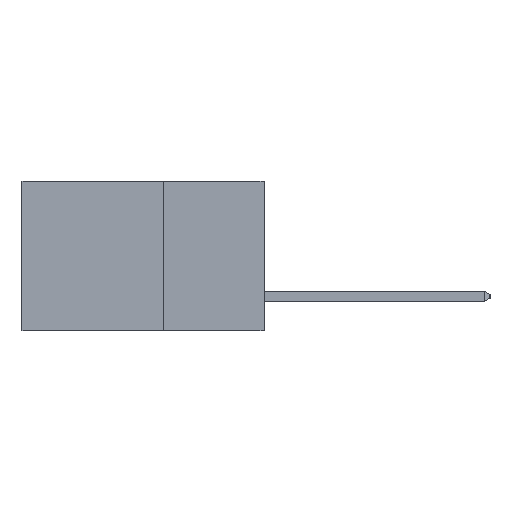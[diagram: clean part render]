
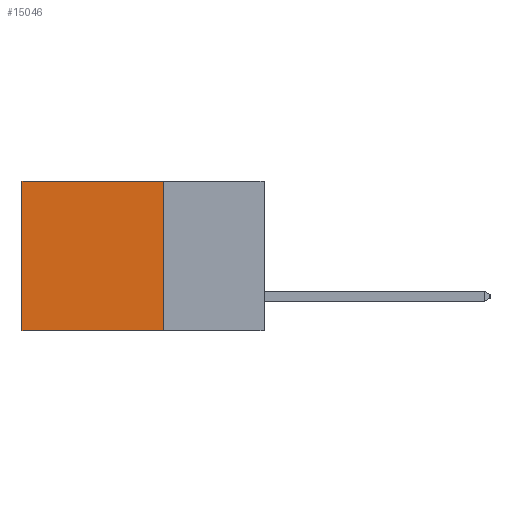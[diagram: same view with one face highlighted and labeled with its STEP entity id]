
A CAD part, left-side view. The second image highlights one B-rep face of the part: STEP entity #15046.
In plain terms, the highlighted planar face has unit normal (-1, 0, 0).
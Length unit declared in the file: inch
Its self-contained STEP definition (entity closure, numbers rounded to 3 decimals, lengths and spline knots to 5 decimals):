
#282 = EDGE_CURVE ( 'NONE', #3886, #5348, #8562, .T. ) ;
#1676 = VECTOR ( 'NONE', #6198, 39.37008 ) ;
#3886 = VERTEX_POINT ( 'NONE', #19722 ) ;
#3986 = ORIENTED_EDGE ( 'NONE', *, *, #11120, .T. ) ;
#5111 = VECTOR ( 'NONE', #10226, 39.37008 ) ;
#5286 = EDGE_CURVE ( 'NONE', #13503, #3886, #6013, .T. ) ;
#5348 = VERTEX_POINT ( 'NONE', #7416 ) ;
#6013 = LINE ( 'NONE', #7579, #1676 ) ;
#6198 = DIRECTION ( 'NONE',  ( 0., 0., -1. ) ) ;
#7416 = CARTESIAN_POINT ( 'NONE',  ( 0.298, 0.6, -0.37 ) ) ;
#7579 = CARTESIAN_POINT ( 'NONE',  ( 0.298, 0.25, 0. ) ) ;
#8562 = LINE ( 'NONE', #20764, #13264 ) ;
#9159 = LINE ( 'NONE', #11643, #13879 ) ;
#9268 = ORIENTED_EDGE ( 'NONE', *, *, #282, .F. ) ;
#9419 = AXIS2_PLACEMENT_3D ( 'NONE', #18428, #20270, #9694 ) ;
#9683 = FACE_OUTER_BOUND ( 'NONE', #10251, .T. ) ;
#9694 = DIRECTION ( 'NONE',  ( 0., 0., -1. ) ) ;
#9998 = LINE ( 'NONE', #10557, #5111 ) ;
#10226 = DIRECTION ( 'NONE',  ( 0., 0., -1. ) ) ;
#10251 = EDGE_LOOP ( 'NONE', ( #3986, #9268, #19847, #18306 ) ) ;
#10557 = CARTESIAN_POINT ( 'NONE',  ( 0.298, 0.6, 0. ) ) ;
#10964 = EDGE_CURVE ( 'NONE', #13503, #13927, #9159, .T. ) ;
#11120 = EDGE_CURVE ( 'NONE', #13927, #5348, #9998, .T. ) ;
#11643 = CARTESIAN_POINT ( 'NONE',  ( 0.298, 0.25, 0. ) ) ;
#11835 = DIRECTION ( 'NONE',  ( 0., 1., 0. ) ) ;
#12919 = CARTESIAN_POINT ( 'NONE',  ( 0.298, 0.25, 0. ) ) ;
#13264 = VECTOR ( 'NONE', #16973, 39.37008 ) ;
#13503 = VERTEX_POINT ( 'NONE', #12919 ) ;
#13879 = VECTOR ( 'NONE', #11835, 39.37008 ) ;
#13927 = VERTEX_POINT ( 'NONE', #19418 ) ;
#15046 = ADVANCED_FACE ( 'NONE', ( #9683 ), #18511, .F. ) ;
#16973 = DIRECTION ( 'NONE',  ( 0., 1., 0. ) ) ;
#18306 = ORIENTED_EDGE ( 'NONE', *, *, #10964, .T. ) ;
#18428 = CARTESIAN_POINT ( 'NONE',  ( 0.298, 0.25, 0. ) ) ;
#18511 = PLANE ( 'NONE',  #9419 ) ;
#19418 = CARTESIAN_POINT ( 'NONE',  ( 0.298, 0.6, 0. ) ) ;
#19722 = CARTESIAN_POINT ( 'NONE',  ( 0.298, 0.25, -0.37 ) ) ;
#19847 = ORIENTED_EDGE ( 'NONE', *, *, #5286, .F. ) ;
#20270 = DIRECTION ( 'NONE',  ( 1., 0., 0. ) ) ;
#20764 = CARTESIAN_POINT ( 'NONE',  ( 0.298, 0.25, -0.37 ) ) ;
